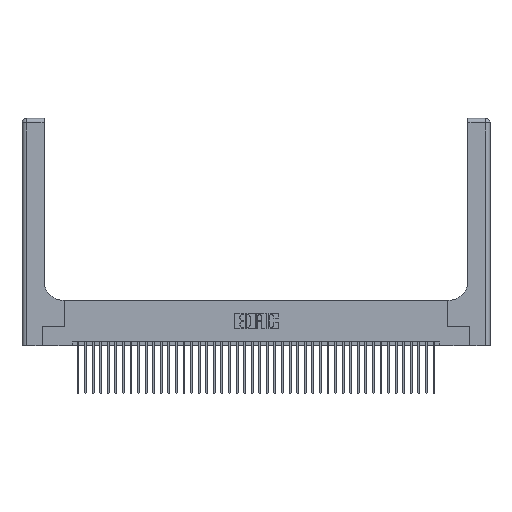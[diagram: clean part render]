
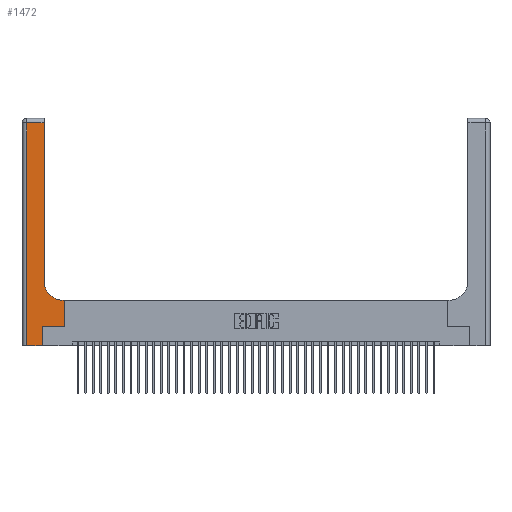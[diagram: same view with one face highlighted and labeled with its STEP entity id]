
A CAD part, top view. The second image highlights one B-rep face of the part: STEP entity #1472.
In plain terms, the highlighted planar face has unit normal (0, 0, 1).
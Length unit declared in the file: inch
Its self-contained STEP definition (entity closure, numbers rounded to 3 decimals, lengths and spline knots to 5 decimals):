
#188 = VECTOR ( 'NONE', #15358, 39.37008 ) ;
#289 = CARTESIAN_POINT ( 'NONE',  ( 0.2915, 3., 0.37 ) ) ;
#733 = VERTEX_POINT ( 'NONE', #11408 ) ;
#1472 = ADVANCED_FACE ( 'NONE', ( #16521 ), #27379, .F. ) ;
#1739 = CARTESIAN_POINT ( 'NONE',  ( 0.06, 0., 0.37 ) ) ;
#1967 = DIRECTION ( 'NONE',  ( -1., 0., 0. ) ) ;
#2039 = DIRECTION ( 'NONE',  ( 0., 1., 0. ) ) ;
#3322 = ORIENTED_EDGE ( 'NONE', *, *, #16216, .T. ) ;
#4568 = VECTOR ( 'NONE', #10068, 39.37008 ) ;
#4827 = VERTEX_POINT ( 'NONE', #40029 ) ;
#4945 = AXIS2_PLACEMENT_3D ( 'NONE', #11146, #17122, #33950 ) ;
#7427 = ORIENTED_EDGE ( 'NONE', *, *, #21618, .T. ) ;
#8140 = CARTESIAN_POINT ( 'NONE',  ( 0., 2.94, 0.37 ) ) ;
#8356 = LINE ( 'NONE', #11932, #188 ) ;
#8716 = ORIENTED_EDGE ( 'NONE', *, *, #28969, .T. ) ;
#8793 = VERTEX_POINT ( 'NONE', #41156 ) ;
#9255 = VECTOR ( 'NONE', #10604, 39.37008 ) ;
#10068 = DIRECTION ( 'NONE',  ( 0., 1., 0. ) ) ;
#10604 = DIRECTION ( 'NONE',  ( 0., -1., 0. ) ) ;
#10758 = CARTESIAN_POINT ( 'NONE',  ( 0.5585, 0.6, 0.37 ) ) ;
#11146 = CARTESIAN_POINT ( 'NONE',  ( 0., 3., 0.37 ) ) ;
#11408 = CARTESIAN_POINT ( 'NONE',  ( 0.5585, 0.25, 0.37 ) ) ;
#11759 = CARTESIAN_POINT ( 'NONE',  ( 0.06, 3., 0.37 ) ) ;
#11932 = CARTESIAN_POINT ( 'NONE',  ( 0., 0., 0.37 ) ) ;
#11944 = CARTESIAN_POINT ( 'NONE',  ( 0.2915, 0.85, 0.37 ) ) ;
#12440 = DIRECTION ( 'NONE',  ( 1., 0., 0. ) ) ;
#12534 = VERTEX_POINT ( 'NONE', #11944 ) ;
#12543 = VERTEX_POINT ( 'NONE', #34601 ) ;
#13698 = VECTOR ( 'NONE', #21348, 39.37008 ) ;
#13791 = ORIENTED_EDGE ( 'NONE', *, *, #20551, .T. ) ;
#14059 = EDGE_CURVE ( 'NONE', #4827, #12534, #23621, .T. ) ;
#15268 = VECTOR ( 'NONE', #34189, 39.37008 ) ;
#15294 = CARTESIAN_POINT ( 'NONE',  ( 0.5415, 0.85, 0.37 ) ) ;
#15358 = DIRECTION ( 'NONE',  ( 1., 0., 0. ) ) ;
#15674 = LINE ( 'NONE', #34081, #20181 ) ;
#15705 = ORIENTED_EDGE ( 'NONE', *, *, #16625, .T. ) ;
#15864 = EDGE_CURVE ( 'NONE', #8793, #12543, #18809, .T. ) ;
#16216 = EDGE_CURVE ( 'NONE', #12534, #8793, #17241, .T. ) ;
#16521 = FACE_OUTER_BOUND ( 'NONE', #35280, .T. ) ;
#16625 = EDGE_CURVE ( 'NONE', #23838, #32278, #17732, .T. ) ;
#17014 = EDGE_CURVE ( 'NONE', #32278, #733, #15674, .T. ) ;
#17122 = DIRECTION ( 'NONE',  ( 0., 0., -1. ) ) ;
#17241 = LINE ( 'NONE', #289, #4568 ) ;
#17732 = LINE ( 'NONE', #21130, #20226 ) ;
#18095 = CARTESIAN_POINT ( 'NONE',  ( 0.5585, 0.25, 0.37 ) ) ;
#18424 = LINE ( 'NONE', #34359, #20944 ) ;
#18809 = LINE ( 'NONE', #8140, #15268 ) ;
#20181 = VECTOR ( 'NONE', #27229, 39.37008 ) ;
#20226 = VECTOR ( 'NONE', #2039, 39.37008 ) ;
#20380 = ORIENTED_EDGE ( 'NONE', *, *, #14059, .T. ) ;
#20551 = EDGE_CURVE ( 'NONE', #12543, #25218, #33690, .T. ) ;
#20944 = VECTOR ( 'NONE', #1967, 39.37008 ) ;
#21130 = CARTESIAN_POINT ( 'NONE',  ( 0.269, 0., 0.37 ) ) ;
#21348 = DIRECTION ( 'NONE',  ( 0., 1., 0. ) ) ;
#21618 = EDGE_CURVE ( 'NONE', #25218, #23838, #8356, .T. ) ;
#21804 = DIRECTION ( 'NONE',  ( 0., 0., -1. ) ) ;
#23621 = CIRCLE ( 'NONE', #39784, 0.25 ) ;
#23838 = VERTEX_POINT ( 'NONE', #28373 ) ;
#24315 = ORIENTED_EDGE ( 'NONE', *, *, #17014, .T. ) ;
#25218 = VERTEX_POINT ( 'NONE', #1739 ) ;
#26994 = ORIENTED_EDGE ( 'NONE', *, *, #15864, .T. ) ;
#27229 = DIRECTION ( 'NONE',  ( 1., 0., 0. ) ) ;
#27379 = PLANE ( 'NONE',  #4945 ) ;
#28129 = VERTEX_POINT ( 'NONE', #10758 ) ;
#28373 = CARTESIAN_POINT ( 'NONE',  ( 0.269, 0., 0.37 ) ) ;
#28969 = EDGE_CURVE ( 'NONE', #28129, #4827, #18424, .T. ) ;
#31468 = ORIENTED_EDGE ( 'NONE', *, *, #40985, .T. ) ;
#32278 = VERTEX_POINT ( 'NONE', #40740 ) ;
#33690 = LINE ( 'NONE', #11759, #9255 ) ;
#33950 = DIRECTION ( 'NONE',  ( -1., 0., 0. ) ) ;
#34081 = CARTESIAN_POINT ( 'NONE',  ( 0.269, 0.25, 0.37 ) ) ;
#34189 = DIRECTION ( 'NONE',  ( -1., 0., 0. ) ) ;
#34359 = CARTESIAN_POINT ( 'NONE',  ( 0.2915, 0.6, 0.37 ) ) ;
#34601 = CARTESIAN_POINT ( 'NONE',  ( 0.06, 2.94, 0.37 ) ) ;
#35122 = LINE ( 'NONE', #18095, #13698 ) ;
#35280 = EDGE_LOOP ( 'NONE', ( #3322, #26994, #13791, #7427, #15705, #24315, #31468, #8716, #20380 ) ) ;
#39784 = AXIS2_PLACEMENT_3D ( 'NONE', #15294, #21804, #12440 ) ;
#40029 = CARTESIAN_POINT ( 'NONE',  ( 0.5415, 0.6, 0.37 ) ) ;
#40740 = CARTESIAN_POINT ( 'NONE',  ( 0.269, 0.25, 0.37 ) ) ;
#40985 = EDGE_CURVE ( 'NONE', #733, #28129, #35122, .T. ) ;
#41156 = CARTESIAN_POINT ( 'NONE',  ( 0.2915, 2.94, 0.37 ) ) ;
